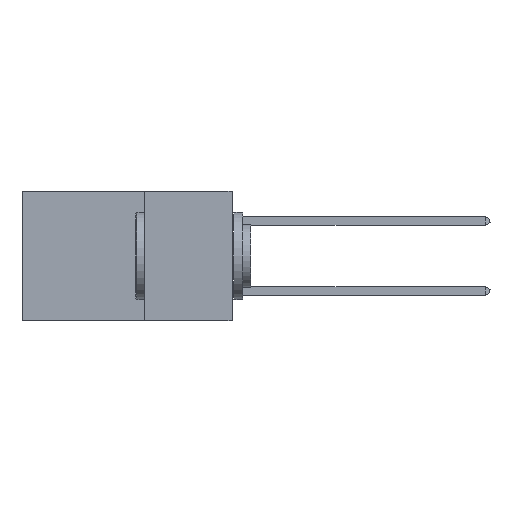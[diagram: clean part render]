
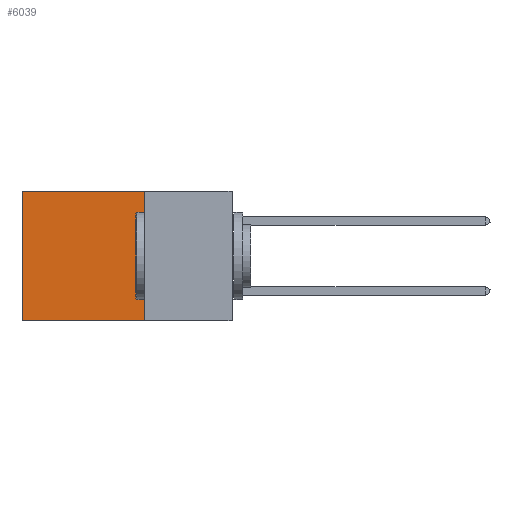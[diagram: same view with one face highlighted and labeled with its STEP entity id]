
A CAD part, left-side view. The second image highlights one B-rep face of the part: STEP entity #6039.
In plain terms, the highlighted planar face has unit normal (-1, 0, 0).
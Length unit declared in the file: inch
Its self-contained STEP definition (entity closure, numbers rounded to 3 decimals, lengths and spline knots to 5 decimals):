
#1156 = LINE ( 'NONE', #21001, #23612 ) ;
#2753 = CARTESIAN_POINT ( 'NONE',  ( 0.2875, 0.25, 0. ) ) ;
#4131 = DIRECTION ( 'NONE',  ( 0., 1., 0. ) ) ;
#4748 = ORIENTED_EDGE ( 'NONE', *, *, #39056, .T. ) ;
#4831 = CARTESIAN_POINT ( 'NONE',  ( 0.2875, 0.25, 0. ) ) ;
#4963 = DIRECTION ( 'NONE',  ( 0., 0., -1. ) ) ;
#5900 = CARTESIAN_POINT ( 'NONE',  ( 0.2875, 0.6, -0.37 ) ) ;
#6039 = ADVANCED_FACE ( 'NONE', ( #29465 ), #14965, .F. ) ;
#8217 = EDGE_CURVE ( 'NONE', #8555, #10621, #19827, .T. ) ;
#8555 = VERTEX_POINT ( 'NONE', #17974 ) ;
#8814 = DIRECTION ( 'NONE',  ( 0., 0., -1. ) ) ;
#8973 = DIRECTION ( 'NONE',  ( 1., 0., 0. ) ) ;
#9038 = VERTEX_POINT ( 'NONE', #26104 ) ;
#10303 = CARTESIAN_POINT ( 'NONE',  ( 0.2875, 0.25, 0. ) ) ;
#10621 = VERTEX_POINT ( 'NONE', #28506 ) ;
#12743 = DIRECTION ( 'NONE',  ( 0., 1., 0. ) ) ;
#14965 = PLANE ( 'NONE',  #33650 ) ;
#17974 = CARTESIAN_POINT ( 'NONE',  ( 0.2875, 0.25, 0. ) ) ;
#19827 = LINE ( 'NONE', #10303, #27858 ) ;
#21001 = CARTESIAN_POINT ( 'NONE',  ( 0.2875, 0.6, 0. ) ) ;
#21456 = LINE ( 'NONE', #4831, #36533 ) ;
#23235 = EDGE_CURVE ( 'NONE', #9038, #31887, #24085, .T. ) ;
#23612 = VECTOR ( 'NONE', #8814, 39.37008 ) ;
#24085 = LINE ( 'NONE', #30815, #32071 ) ;
#26104 = CARTESIAN_POINT ( 'NONE',  ( 0.2875, 0.25, -0.37 ) ) ;
#27858 = VECTOR ( 'NONE', #4131, 39.37008 ) ;
#28506 = CARTESIAN_POINT ( 'NONE',  ( 0.2875, 0.6, 0. ) ) ;
#28811 = ORIENTED_EDGE ( 'NONE', *, *, #8217, .T. ) ;
#29465 = FACE_OUTER_BOUND ( 'NONE', #31371, .T. ) ;
#30112 = DIRECTION ( 'NONE',  ( 0., 0., -1. ) ) ;
#30815 = CARTESIAN_POINT ( 'NONE',  ( 0.2875, 0.25, -0.37 ) ) ;
#31371 = EDGE_LOOP ( 'NONE', ( #4748, #32975, #37311, #28811 ) ) ;
#31887 = VERTEX_POINT ( 'NONE', #5900 ) ;
#32071 = VECTOR ( 'NONE', #12743, 39.37008 ) ;
#32975 = ORIENTED_EDGE ( 'NONE', *, *, #23235, .F. ) ;
#33650 = AXIS2_PLACEMENT_3D ( 'NONE', #2753, #8973, #30112 ) ;
#36533 = VECTOR ( 'NONE', #4963, 39.37008 ) ;
#36697 = EDGE_CURVE ( 'NONE', #8555, #9038, #21456, .T. ) ;
#37311 = ORIENTED_EDGE ( 'NONE', *, *, #36697, .F. ) ;
#39056 = EDGE_CURVE ( 'NONE', #10621, #31887, #1156, .T. ) ;
